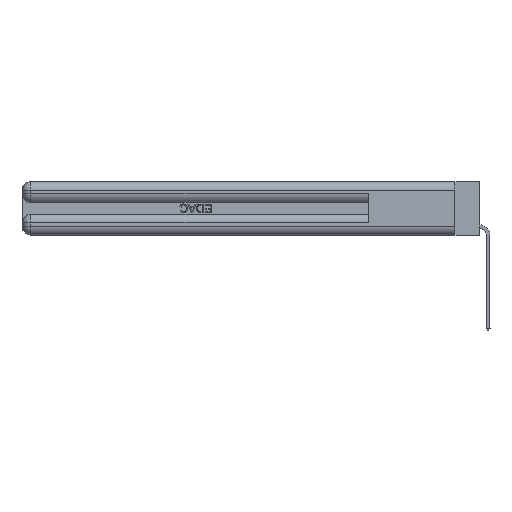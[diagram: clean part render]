
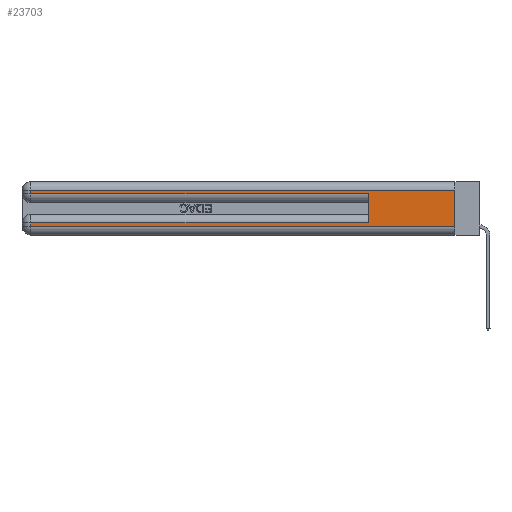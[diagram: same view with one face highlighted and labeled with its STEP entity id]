
A CAD part, left-side view. The second image highlights one B-rep face of the part: STEP entity #23703.
In plain terms, the highlighted planar face has unit normal (-1, 0, 0).
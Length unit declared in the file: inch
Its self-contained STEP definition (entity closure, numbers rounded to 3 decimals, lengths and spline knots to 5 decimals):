
#22 = EDGE_CURVE ( 'NONE', #11168, #13561, #765, .T. ) ;
#539 = LINE ( 'NONE', #19761, #1362 ) ;
#574 = LINE ( 'NONE', #33246, #20310 ) ;
#765 = LINE ( 'NONE', #23967, #14398 ) ;
#955 = VERTEX_POINT ( 'NONE', #25939 ) ;
#976 = EDGE_CURVE ( 'NONE', #955, #6534, #31775, .T. ) ;
#1059 = EDGE_CURVE ( 'NONE', #6534, #21290, #30176, .T. ) ;
#1069 = CARTESIAN_POINT ( 'NONE',  ( 0., 0., 0.06 ) ) ;
#1362 = VECTOR ( 'NONE', #27490, 39.37008 ) ;
#1496 = ORIENTED_EDGE ( 'NONE', *, *, #1059, .T. ) ;
#2055 = LINE ( 'NONE', #13198, #8897 ) ;
#2100 = VERTEX_POINT ( 'NONE', #21707 ) ;
#2224 = CARTESIAN_POINT ( 'NONE',  ( 0., 0., 0.31 ) ) ;
#2437 = CARTESIAN_POINT ( 'NONE',  ( 0., 2.94, 0.31 ) ) ;
#3020 = DIRECTION ( 'NONE',  ( 0., 0., 1. ) ) ;
#3397 = EDGE_CURVE ( 'NONE', #2100, #955, #574, .T. ) ;
#3578 = CARTESIAN_POINT ( 'NONE',  ( 0., 2.94, 0.285 ) ) ;
#3682 = VERTEX_POINT ( 'NONE', #3578 ) ;
#3847 = EDGE_CURVE ( 'NONE', #3682, #11678, #539, .T. ) ;
#4285 = ORIENTED_EDGE ( 'NONE', *, *, #3847, .T. ) ;
#4923 = DIRECTION ( 'NONE',  ( 0., 1., 0. ) ) ;
#4992 = CARTESIAN_POINT ( 'NONE',  ( 0., 0.6, 0.285 ) ) ;
#5092 = ORIENTED_EDGE ( 'NONE', *, *, #27629, .F. ) ;
#6534 = VERTEX_POINT ( 'NONE', #23813 ) ;
#6747 = DIRECTION ( 'NONE',  ( 0., 0., -1. ) ) ;
#7076 = AXIS2_PLACEMENT_3D ( 'NONE', #23576, #10771, #28911 ) ;
#7820 = FACE_OUTER_BOUND ( 'NONE', #11308, .T. ) ;
#8210 = PLANE ( 'NONE',  #7076 ) ;
#8497 = DIRECTION ( 'NONE',  ( 0., 1., 0. ) ) ;
#8897 = VECTOR ( 'NONE', #3020, 39.37008 ) ;
#9501 = ORIENTED_EDGE ( 'NONE', *, *, #22136, .T. ) ;
#10771 = DIRECTION ( 'NONE',  ( 1., 0., 0. ) ) ;
#11168 = VERTEX_POINT ( 'NONE', #2224 ) ;
#11308 = EDGE_LOOP ( 'NONE', ( #24462, #14709, #9501, #4285, #5092, #12690, #21242, #1496 ) ) ;
#11678 = VERTEX_POINT ( 'NONE', #4992 ) ;
#12690 = ORIENTED_EDGE ( 'NONE', *, *, #3397, .T. ) ;
#13198 = CARTESIAN_POINT ( 'NONE',  ( 0., 0.6, 0.145 ) ) ;
#13561 = VERTEX_POINT ( 'NONE', #2437 ) ;
#14398 = VECTOR ( 'NONE', #8497, 39.37008 ) ;
#14709 = ORIENTED_EDGE ( 'NONE', *, *, #22, .T. ) ;
#16825 = CARTESIAN_POINT ( 'NONE',  ( 0., 2.94, 0.37 ) ) ;
#17780 = EDGE_CURVE ( 'NONE', #11168, #21290, #19862, .T. ) ;
#19761 = CARTESIAN_POINT ( 'NONE',  ( 0., 0., 0.285 ) ) ;
#19862 = LINE ( 'NONE', #21115, #25951 ) ;
#20245 = DIRECTION ( 'NONE',  ( 0., 0., -1. ) ) ;
#20310 = VECTOR ( 'NONE', #4923, 39.37008 ) ;
#21115 = CARTESIAN_POINT ( 'NONE',  ( 0., 0., 0.37 ) ) ;
#21242 = ORIENTED_EDGE ( 'NONE', *, *, #976, .T. ) ;
#21255 = VECTOR ( 'NONE', #20245, 39.37008 ) ;
#21290 = VERTEX_POINT ( 'NONE', #1069 ) ;
#21707 = CARTESIAN_POINT ( 'NONE',  ( 0., 0.6, 0.085 ) ) ;
#22136 = EDGE_CURVE ( 'NONE', #13561, #3682, #27335, .T. ) ;
#23576 = CARTESIAN_POINT ( 'NONE',  ( 0., 0., 0.37 ) ) ;
#23703 = ADVANCED_FACE ( 'NONE', ( #7820 ), #8210, .F. ) ;
#23745 = DIRECTION ( 'NONE',  ( 0., 0., -1. ) ) ;
#23813 = CARTESIAN_POINT ( 'NONE',  ( 0., 2.94, 0.06 ) ) ;
#23967 = CARTESIAN_POINT ( 'NONE',  ( 0., 0., 0.31 ) ) ;
#24462 = ORIENTED_EDGE ( 'NONE', *, *, #17780, .F. ) ;
#24897 = VECTOR ( 'NONE', #6747, 39.37008 ) ;
#25939 = CARTESIAN_POINT ( 'NONE',  ( 0., 2.94, 0.085 ) ) ;
#25951 = VECTOR ( 'NONE', #23745, 39.37008 ) ;
#27335 = LINE ( 'NONE', #33129, #21255 ) ;
#27490 = DIRECTION ( 'NONE',  ( 0., -1., 0. ) ) ;
#27629 = EDGE_CURVE ( 'NONE', #2100, #11678, #2055, .T. ) ;
#28547 = DIRECTION ( 'NONE',  ( 0., -1., 0. ) ) ;
#28698 = CARTESIAN_POINT ( 'NONE',  ( 0., 0., 0.06 ) ) ;
#28911 = DIRECTION ( 'NONE',  ( 0., 0., -1. ) ) ;
#30176 = LINE ( 'NONE', #28698, #32554 ) ;
#31775 = LINE ( 'NONE', #16825, #24897 ) ;
#32554 = VECTOR ( 'NONE', #28547, 39.37008 ) ;
#33129 = CARTESIAN_POINT ( 'NONE',  ( 0., 2.94, 0.37 ) ) ;
#33246 = CARTESIAN_POINT ( 'NONE',  ( 0., 0., 0.085 ) ) ;
